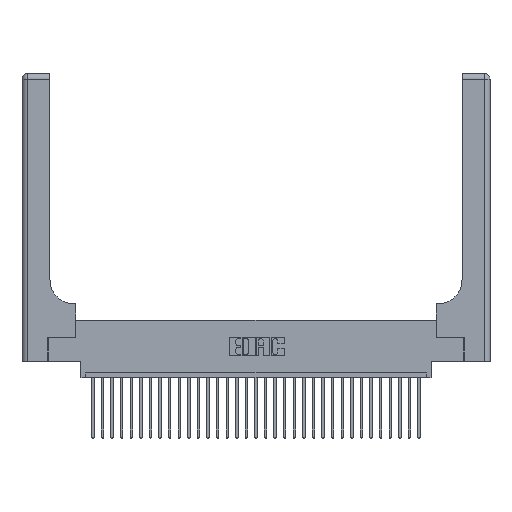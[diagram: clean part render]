
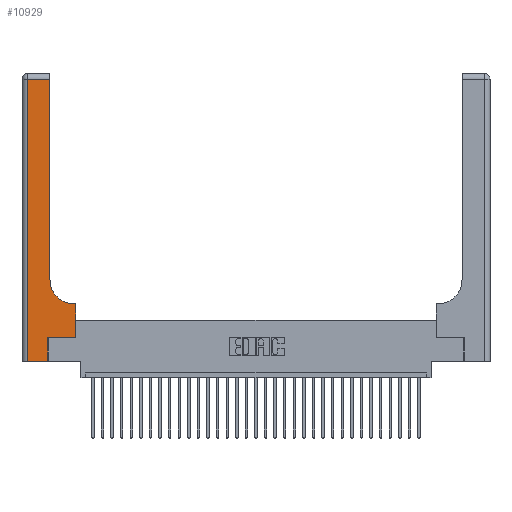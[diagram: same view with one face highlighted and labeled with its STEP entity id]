
A CAD part, top view. The second image highlights one B-rep face of the part: STEP entity #10929.
In plain terms, the highlighted planar face has unit normal (0, 0, 1).
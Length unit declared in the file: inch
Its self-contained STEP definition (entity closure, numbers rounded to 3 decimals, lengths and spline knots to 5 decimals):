
#231 = PLANE ( 'NONE',  #25694 ) ;
#407 = CARTESIAN_POINT ( 'NONE',  ( 0.06, 3., 0.37 ) ) ;
#537 = CARTESIAN_POINT ( 'NONE',  ( 0.5415, 0.85, 0.37 ) ) ;
#576 = VERTEX_POINT ( 'NONE', #3905 ) ;
#813 = CARTESIAN_POINT ( 'NONE',  ( 0.2915, 0.85, 0.37 ) ) ;
#1273 = EDGE_CURVE ( 'NONE', #29177, #15767, #28962, .T. ) ;
#1290 = EDGE_CURVE ( 'NONE', #28332, #2293, #17659, .T. ) ;
#2293 = VERTEX_POINT ( 'NONE', #2621 ) ;
#2412 = VECTOR ( 'NONE', #13106, 39.37008 ) ;
#2549 = EDGE_CURVE ( 'NONE', #2293, #28072, #32504, .T. ) ;
#2621 = CARTESIAN_POINT ( 'NONE',  ( 0.5585, 0.25, 0.37 ) ) ;
#2627 = LINE ( 'NONE', #15850, #26592 ) ;
#2748 = DIRECTION ( 'NONE',  ( -1., 0., 0. ) ) ;
#3905 = CARTESIAN_POINT ( 'NONE',  ( 0.06, 0., 0.37 ) ) ;
#4203 = CIRCLE ( 'NONE', #26941, 0.25 ) ;
#4815 = DIRECTION ( 'NONE',  ( 1., 0., 0. ) ) ;
#4943 = VERTEX_POINT ( 'NONE', #26276 ) ;
#6217 = CARTESIAN_POINT ( 'NONE',  ( 0.269, 0., 0.37 ) ) ;
#7916 = DIRECTION ( 'NONE',  ( -1., 0., 0. ) ) ;
#8242 = DIRECTION ( 'NONE',  ( 0., 0., -1. ) ) ;
#9895 = EDGE_LOOP ( 'NONE', ( #19258, #21329, #31129, #27913, #19335, #16775, #28410, #20787, #22106 ) ) ;
#10127 = EDGE_CURVE ( 'NONE', #21239, #28332, #2627, .T. ) ;
#10396 = LINE ( 'NONE', #24947, #14365 ) ;
#10586 = CARTESIAN_POINT ( 'NONE',  ( 0.269, 0.25, 0.37 ) ) ;
#10877 = VECTOR ( 'NONE', #7916, 39.37008 ) ;
#10929 = ADVANCED_FACE ( 'NONE', ( #30131 ), #231, .F. ) ;
#10937 = VECTOR ( 'NONE', #27342, 39.37008 ) ;
#11234 = VECTOR ( 'NONE', #17609, 39.37008 ) ;
#11715 = VECTOR ( 'NONE', #25504, 39.37008 ) ;
#13106 = DIRECTION ( 'NONE',  ( 0., -1., 0. ) ) ;
#13107 = DIRECTION ( 'NONE',  ( 0., 1., 0. ) ) ;
#13145 = DIRECTION ( 'NONE',  ( 1., 0., 0. ) ) ;
#14365 = VECTOR ( 'NONE', #4815, 39.37008 ) ;
#14547 = CARTESIAN_POINT ( 'NONE',  ( 0., 2.94, 0.37 ) ) ;
#15042 = EDGE_CURVE ( 'NONE', #28072, #19749, #30935, .T. ) ;
#15767 = VERTEX_POINT ( 'NONE', #24606 ) ;
#15850 = CARTESIAN_POINT ( 'NONE',  ( 0.269, 0., 0.37 ) ) ;
#16775 = ORIENTED_EDGE ( 'NONE', *, *, #1290, .T. ) ;
#17536 = CARTESIAN_POINT ( 'NONE',  ( 0.2915, 0.6, 0.37 ) ) ;
#17609 = DIRECTION ( 'NONE',  ( 0., 1., 0. ) ) ;
#17659 = LINE ( 'NONE', #10586, #31760 ) ;
#17881 = CARTESIAN_POINT ( 'NONE',  ( 0., 3., 0.37 ) ) ;
#17899 = CARTESIAN_POINT ( 'NONE',  ( 0.5585, 0.6, 0.37 ) ) ;
#18212 = EDGE_CURVE ( 'NONE', #4943, #576, #21275, .T. ) ;
#19258 = ORIENTED_EDGE ( 'NONE', *, *, #1273, .T. ) ;
#19335 = ORIENTED_EDGE ( 'NONE', *, *, #10127, .T. ) ;
#19749 = VERTEX_POINT ( 'NONE', #26311 ) ;
#20478 = CARTESIAN_POINT ( 'NONE',  ( 0.2915, 3., 0.37 ) ) ;
#20787 = ORIENTED_EDGE ( 'NONE', *, *, #15042, .T. ) ;
#21079 = EDGE_CURVE ( 'NONE', #19749, #29177, #4203, .T. ) ;
#21239 = VERTEX_POINT ( 'NONE', #6217 ) ;
#21275 = LINE ( 'NONE', #407, #2412 ) ;
#21329 = ORIENTED_EDGE ( 'NONE', *, *, #31979, .T. ) ;
#22106 = ORIENTED_EDGE ( 'NONE', *, *, #21079, .T. ) ;
#22743 = CARTESIAN_POINT ( 'NONE',  ( 0.5585, 0.25, 0.37 ) ) ;
#23124 = DIRECTION ( 'NONE',  ( 0., 0., -1. ) ) ;
#24606 = CARTESIAN_POINT ( 'NONE',  ( 0.2915, 2.94, 0.37 ) ) ;
#24947 = CARTESIAN_POINT ( 'NONE',  ( 0., 0., 0.37 ) ) ;
#25504 = DIRECTION ( 'NONE',  ( 0., 1., 0. ) ) ;
#25694 = AXIS2_PLACEMENT_3D ( 'NONE', #17881, #23124, #2748 ) ;
#26276 = CARTESIAN_POINT ( 'NONE',  ( 0.06, 2.94, 0.37 ) ) ;
#26311 = CARTESIAN_POINT ( 'NONE',  ( 0.5415, 0.6, 0.37 ) ) ;
#26592 = VECTOR ( 'NONE', #13107, 39.37008 ) ;
#26941 = AXIS2_PLACEMENT_3D ( 'NONE', #537, #8242, #27891 ) ;
#27014 = LINE ( 'NONE', #14547, #10937 ) ;
#27342 = DIRECTION ( 'NONE',  ( -1., 0., 0. ) ) ;
#27891 = DIRECTION ( 'NONE',  ( 1., 0., 0. ) ) ;
#27913 = ORIENTED_EDGE ( 'NONE', *, *, #30674, .T. ) ;
#28072 = VERTEX_POINT ( 'NONE', #17899 ) ;
#28236 = CARTESIAN_POINT ( 'NONE',  ( 0.269, 0.25, 0.37 ) ) ;
#28332 = VERTEX_POINT ( 'NONE', #28236 ) ;
#28410 = ORIENTED_EDGE ( 'NONE', *, *, #2549, .T. ) ;
#28962 = LINE ( 'NONE', #20478, #11715 ) ;
#29177 = VERTEX_POINT ( 'NONE', #813 ) ;
#30131 = FACE_OUTER_BOUND ( 'NONE', #9895, .T. ) ;
#30674 = EDGE_CURVE ( 'NONE', #576, #21239, #10396, .T. ) ;
#30935 = LINE ( 'NONE', #17536, #10877 ) ;
#31129 = ORIENTED_EDGE ( 'NONE', *, *, #18212, .T. ) ;
#31760 = VECTOR ( 'NONE', #13145, 39.37008 ) ;
#31979 = EDGE_CURVE ( 'NONE', #15767, #4943, #27014, .T. ) ;
#32504 = LINE ( 'NONE', #22743, #11234 ) ;
